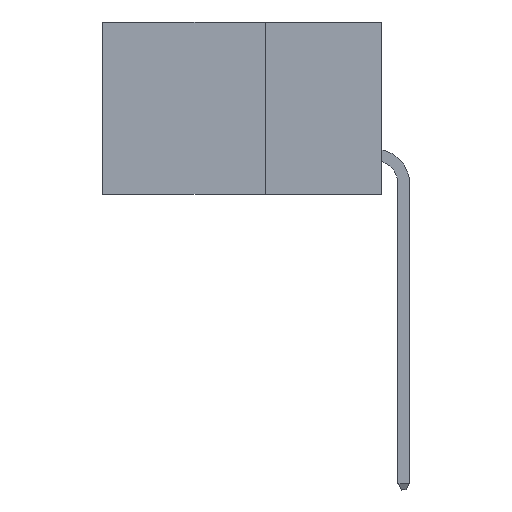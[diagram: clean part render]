
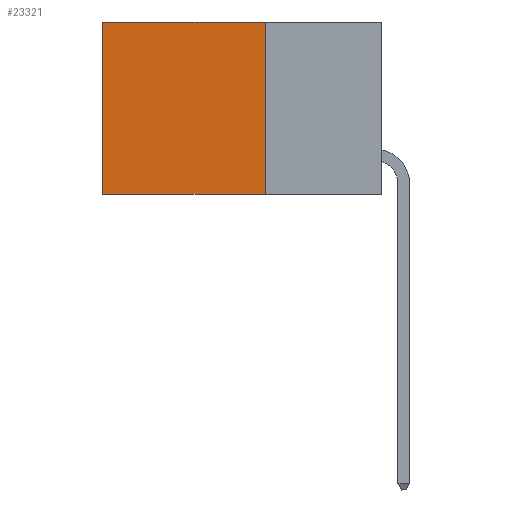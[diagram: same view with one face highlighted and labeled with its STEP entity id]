
A CAD part, left-side view. The second image highlights one B-rep face of the part: STEP entity #23321.
In plain terms, the highlighted planar face has unit normal (-1, 0, 0).
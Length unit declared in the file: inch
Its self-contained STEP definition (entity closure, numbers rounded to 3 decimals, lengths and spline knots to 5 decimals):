
#722 = DIRECTION ( 'NONE',  ( 0., 1., 0. ) ) ;
#1331 = ORIENTED_EDGE ( 'NONE', *, *, #10884, .T. ) ;
#1441 = CARTESIAN_POINT ( 'NONE',  ( 0.2875, 0.25, 0. ) ) ;
#1766 = CARTESIAN_POINT ( 'NONE',  ( 0.2875, 0.6, 0. ) ) ;
#1875 = VERTEX_POINT ( 'NONE', #1441 ) ;
#2004 = EDGE_LOOP ( 'NONE', ( #1331, #7849, #6758, #16681 ) ) ;
#2607 = LINE ( 'NONE', #19703, #12363 ) ;
#3430 = CARTESIAN_POINT ( 'NONE',  ( 0.2875, 0.6, 0. ) ) ;
#4384 = LINE ( 'NONE', #15120, #22655 ) ;
#4540 = LINE ( 'NONE', #3430, #18628 ) ;
#5282 = CARTESIAN_POINT ( 'NONE',  ( 0.2875, 0.25, -0.37 ) ) ;
#6758 = ORIENTED_EDGE ( 'NONE', *, *, #13950, .F. ) ;
#7063 = DIRECTION ( 'NONE',  ( 0., 0., -1. ) ) ;
#7849 = ORIENTED_EDGE ( 'NONE', *, *, #9209, .F. ) ;
#8529 = CARTESIAN_POINT ( 'NONE',  ( 0.2875, 0.6, -0.37 ) ) ;
#8706 = DIRECTION ( 'NONE',  ( 0., 1., 0. ) ) ;
#9209 = EDGE_CURVE ( 'NONE', #21925, #16732, #2607, .T. ) ;
#10849 = FACE_OUTER_BOUND ( 'NONE', #2004, .T. ) ;
#10884 = EDGE_CURVE ( 'NONE', #23294, #16732, #4540, .T. ) ;
#12363 = VECTOR ( 'NONE', #8706, 39.37008 ) ;
#12885 = DIRECTION ( 'NONE',  ( 0., 0., -1. ) ) ;
#13390 = EDGE_CURVE ( 'NONE', #1875, #23294, #17086, .T. ) ;
#13950 = EDGE_CURVE ( 'NONE', #1875, #21925, #4384, .T. ) ;
#15120 = CARTESIAN_POINT ( 'NONE',  ( 0.2875, 0.25, 0. ) ) ;
#16681 = ORIENTED_EDGE ( 'NONE', *, *, #13390, .T. ) ;
#16718 = AXIS2_PLACEMENT_3D ( 'NONE', #22079, #21936, #12885 ) ;
#16732 = VERTEX_POINT ( 'NONE', #8529 ) ;
#17086 = LINE ( 'NONE', #22627, #21639 ) ;
#18628 = VECTOR ( 'NONE', #7063, 39.37008 ) ;
#19096 = DIRECTION ( 'NONE',  ( 0., 0., -1. ) ) ;
#19703 = CARTESIAN_POINT ( 'NONE',  ( 0.2875, 0.25, -0.37 ) ) ;
#20373 = PLANE ( 'NONE',  #16718 ) ;
#21639 = VECTOR ( 'NONE', #722, 39.37008 ) ;
#21925 = VERTEX_POINT ( 'NONE', #5282 ) ;
#21936 = DIRECTION ( 'NONE',  ( 1., 0., 0. ) ) ;
#22079 = CARTESIAN_POINT ( 'NONE',  ( 0.2875, 0.25, 0. ) ) ;
#22627 = CARTESIAN_POINT ( 'NONE',  ( 0.2875, 0.25, 0. ) ) ;
#22655 = VECTOR ( 'NONE', #19096, 39.37008 ) ;
#23294 = VERTEX_POINT ( 'NONE', #1766 ) ;
#23321 = ADVANCED_FACE ( 'NONE', ( #10849 ), #20373, .F. ) ;
